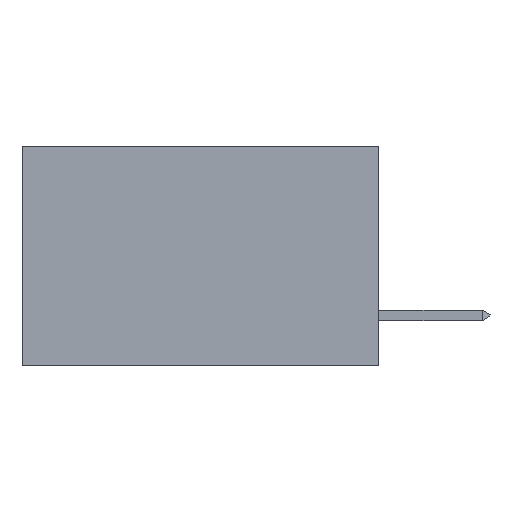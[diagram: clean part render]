
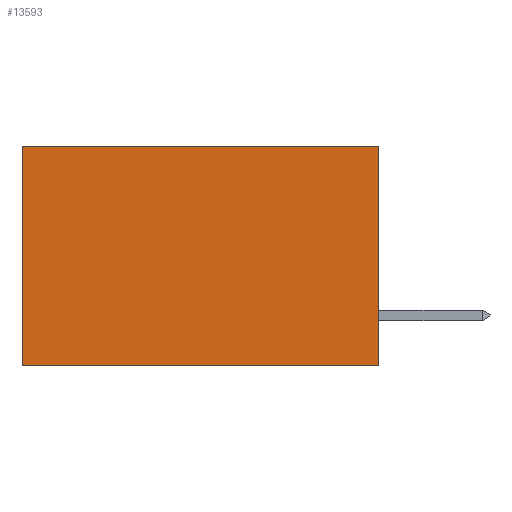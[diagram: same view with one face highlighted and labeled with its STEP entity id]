
A CAD part, left-side view. The second image highlights one B-rep face of the part: STEP entity #13593.
In plain terms, the highlighted planar face has unit normal (-1, 0, 0).
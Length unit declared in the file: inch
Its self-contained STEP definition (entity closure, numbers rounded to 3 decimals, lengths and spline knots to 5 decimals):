
#527 = CARTESIAN_POINT ( 'NONE',  ( 0.2615, 0., -0.37 ) ) ;
#2341 = EDGE_CURVE ( 'NONE', #13123, #11331, #20198, .T. ) ;
#2537 = DIRECTION ( 'NONE',  ( 0., 0., -1. ) ) ;
#3059 = PLANE ( 'NONE',  #12726 ) ;
#4686 = CARTESIAN_POINT ( 'NONE',  ( 0.2615, 0.6, 0. ) ) ;
#5524 = DIRECTION ( 'NONE',  ( 0., 0., -1. ) ) ;
#6541 = VECTOR ( 'NONE', #19804, 39.37008 ) ;
#7109 = CARTESIAN_POINT ( 'NONE',  ( 0.2615, 0., -0.37 ) ) ;
#7177 = EDGE_CURVE ( 'NONE', #13123, #10606, #11813, .T. ) ;
#8131 = ORIENTED_EDGE ( 'NONE', *, *, #2341, .T. ) ;
#8589 = CARTESIAN_POINT ( 'NONE',  ( 0.2615, 0., 0. ) ) ;
#9043 = ORIENTED_EDGE ( 'NONE', *, *, #7177, .F. ) ;
#9461 = VECTOR ( 'NONE', #5524, 39.37008 ) ;
#10606 = VERTEX_POINT ( 'NONE', #7109 ) ;
#10969 = DIRECTION ( 'NONE',  ( 1., 0., 0. ) ) ;
#11213 = CARTESIAN_POINT ( 'NONE',  ( 0.2615, 0.6, -0.37 ) ) ;
#11239 = VECTOR ( 'NONE', #23499, 39.37008 ) ;
#11331 = VERTEX_POINT ( 'NONE', #4686 ) ;
#11468 = EDGE_LOOP ( 'NONE', ( #22561, #20244, #9043, #8131 ) ) ;
#11783 = LINE ( 'NONE', #15634, #11239 ) ;
#11813 = LINE ( 'NONE', #527, #24012 ) ;
#11940 = CARTESIAN_POINT ( 'NONE',  ( 0.2615, 0., 0. ) ) ;
#12379 = CARTESIAN_POINT ( 'NONE',  ( 0.2615, 0., -0.37 ) ) ;
#12726 = AXIS2_PLACEMENT_3D ( 'NONE', #12379, #10969, #2537 ) ;
#12883 = FACE_OUTER_BOUND ( 'NONE', #11468, .T. ) ;
#13123 = VERTEX_POINT ( 'NONE', #8589 ) ;
#13593 = ADVANCED_FACE ( 'NONE', ( #12883 ), #3059, .F. ) ;
#13694 = EDGE_CURVE ( 'NONE', #11331, #24309, #23181, .T. ) ;
#15634 = CARTESIAN_POINT ( 'NONE',  ( 0.2615, 0., -0.37 ) ) ;
#15924 = DIRECTION ( 'NONE',  ( 0., 0., -1. ) ) ;
#19039 = EDGE_CURVE ( 'NONE', #10606, #24309, #11783, .T. ) ;
#19804 = DIRECTION ( 'NONE',  ( 0., 1., 0. ) ) ;
#20198 = LINE ( 'NONE', #11940, #6541 ) ;
#20244 = ORIENTED_EDGE ( 'NONE', *, *, #19039, .F. ) ;
#22561 = ORIENTED_EDGE ( 'NONE', *, *, #13694, .T. ) ;
#22611 = CARTESIAN_POINT ( 'NONE',  ( 0.2615, 0.6, -0.37 ) ) ;
#23181 = LINE ( 'NONE', #11213, #9461 ) ;
#23499 = DIRECTION ( 'NONE',  ( 0., 1., 0. ) ) ;
#24012 = VECTOR ( 'NONE', #15924, 39.37008 ) ;
#24309 = VERTEX_POINT ( 'NONE', #22611 ) ;
